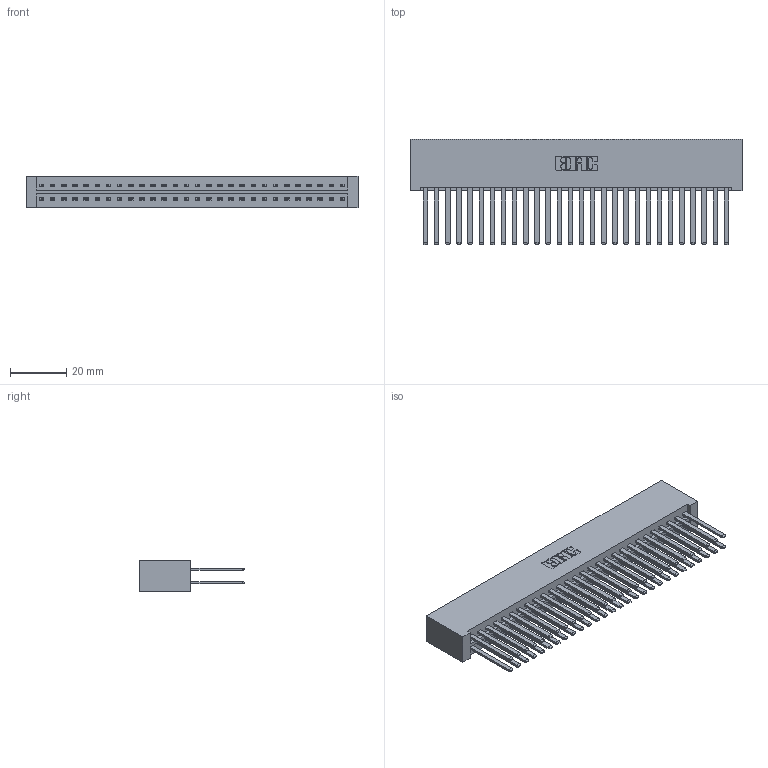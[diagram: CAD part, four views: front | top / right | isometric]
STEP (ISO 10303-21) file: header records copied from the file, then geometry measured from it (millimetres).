
FILE_DESCRIPTION (( 'STEP AP203' ), '1' );
FILE_NAME ('336-056-541-801.STEP', '2020-08-08T00:24:44', ( '' ), ( '' ), 'SwSTEP 2.0', 'SolidWorks 2020', '' );
FILE_SCHEMA (( 'CONFIG_CONTROL_DESIGN' ));
Length unit declared in the file: inch
Products named in the file (3): 336-290-001_336-290-541; 336 Part_Lugless; 336-056-541-801
Assembly tree (57 placements, depth 2):
  336-056-541-801
    336 Part_Lugless
    336-290-001_336-290-541  x56
Bounding box: 118.06 x 37.34 x 11.1 mm (x, y, z)
Volume: 19467.9 mm3; surface area: 24824.1 mm2
Topology: 57 solids, 57 shells, 2458 faces, 7399 edges, 4894 vertices
Faces by surface type: plane 1522, cylinder 936
Entity records: 22962 total; most frequent: CARTESIAN_POINT 3961, ORIENTED_EDGE 3798, DIRECTION 3291, EDGE_CURVE 1899, VECTOR 1775, LINE 1775, VERTEX_POINT 1264, AXIS2_PLACEMENT_3D 758
